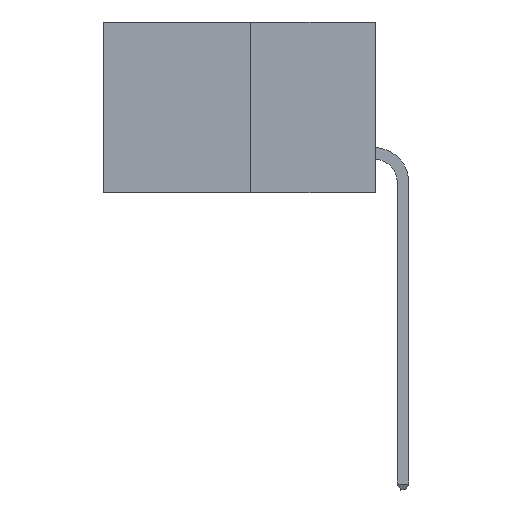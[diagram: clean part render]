
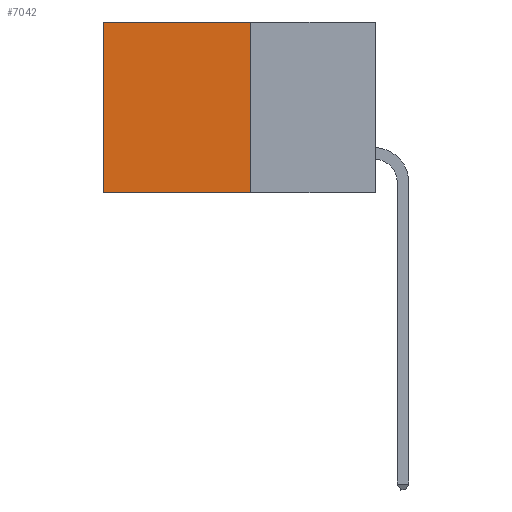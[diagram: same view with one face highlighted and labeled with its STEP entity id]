
A CAD part, left-side view. The second image highlights one B-rep face of the part: STEP entity #7042.
In plain terms, the highlighted planar face has unit normal (-1, 0, 0).
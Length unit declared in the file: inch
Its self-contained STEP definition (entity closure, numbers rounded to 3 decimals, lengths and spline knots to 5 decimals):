
#363 = DIRECTION ( 'NONE',  ( 1., 0., 0. ) ) ;
#536 = ORIENTED_EDGE ( 'NONE', *, *, #11281, .F. ) ;
#810 = VECTOR ( 'NONE', #10301, 39.37008 ) ;
#1116 = LINE ( 'NONE', #5124, #810 ) ;
#1392 = CARTESIAN_POINT ( 'NONE',  ( 0.277, 0.27, -0.37 ) ) ;
#1633 = ORIENTED_EDGE ( 'NONE', *, *, #7525, .F. ) ;
#1771 = ORIENTED_EDGE ( 'NONE', *, *, #6786, .T. ) ;
#2165 = VERTEX_POINT ( 'NONE', #8857 ) ;
#2300 = AXIS2_PLACEMENT_3D ( 'NONE', #6705, #363, #3171 ) ;
#2447 = VECTOR ( 'NONE', #3993, 39.37008 ) ;
#2738 = LINE ( 'NONE', #1392, #4873 ) ;
#3171 = DIRECTION ( 'NONE',  ( 0., 0., -1. ) ) ;
#3812 = CARTESIAN_POINT ( 'NONE',  ( 0.277, 0.27, -0.37 ) ) ;
#3993 = DIRECTION ( 'NONE',  ( 0., 1., 0. ) ) ;
#4312 = LINE ( 'NONE', #8366, #2447 ) ;
#4428 = VERTEX_POINT ( 'NONE', #6659 ) ;
#4568 = VERTEX_POINT ( 'NONE', #9080 ) ;
#4698 = LINE ( 'NONE', #3812, #9067 ) ;
#4873 = VECTOR ( 'NONE', #11172, 39.37008 ) ;
#5000 = FACE_OUTER_BOUND ( 'NONE', #8306, .T. ) ;
#5124 = CARTESIAN_POINT ( 'NONE',  ( 0.277, 0.59, -0.37 ) ) ;
#6659 = CARTESIAN_POINT ( 'NONE',  ( 0.277, 0.27, 0. ) ) ;
#6705 = CARTESIAN_POINT ( 'NONE',  ( 0.277, 0.27, -0.37 ) ) ;
#6775 = PLANE ( 'NONE',  #2300 ) ;
#6786 = EDGE_CURVE ( 'NONE', #2165, #4568, #1116, .T. ) ;
#6876 = VERTEX_POINT ( 'NONE', #10934 ) ;
#7042 = ADVANCED_FACE ( 'NONE', ( #5000 ), #6775, .F. ) ;
#7525 = EDGE_CURVE ( 'NONE', #6876, #4568, #2738, .T. ) ;
#8306 = EDGE_LOOP ( 'NONE', ( #1771, #1633, #536, #11167 ) ) ;
#8366 = CARTESIAN_POINT ( 'NONE',  ( 0.277, 0.27, 0. ) ) ;
#8857 = CARTESIAN_POINT ( 'NONE',  ( 0.277, 0.59, 0. ) ) ;
#9067 = VECTOR ( 'NONE', #10828, 39.37008 ) ;
#9080 = CARTESIAN_POINT ( 'NONE',  ( 0.277, 0.59, -0.37 ) ) ;
#10301 = DIRECTION ( 'NONE',  ( 0., 0., -1. ) ) ;
#10700 = EDGE_CURVE ( 'NONE', #4428, #2165, #4312, .T. ) ;
#10828 = DIRECTION ( 'NONE',  ( 0., 0., -1. ) ) ;
#10934 = CARTESIAN_POINT ( 'NONE',  ( 0.277, 0.27, -0.37 ) ) ;
#11167 = ORIENTED_EDGE ( 'NONE', *, *, #10700, .T. ) ;
#11172 = DIRECTION ( 'NONE',  ( 0., 1., 0. ) ) ;
#11281 = EDGE_CURVE ( 'NONE', #4428, #6876, #4698, .T. ) ;
